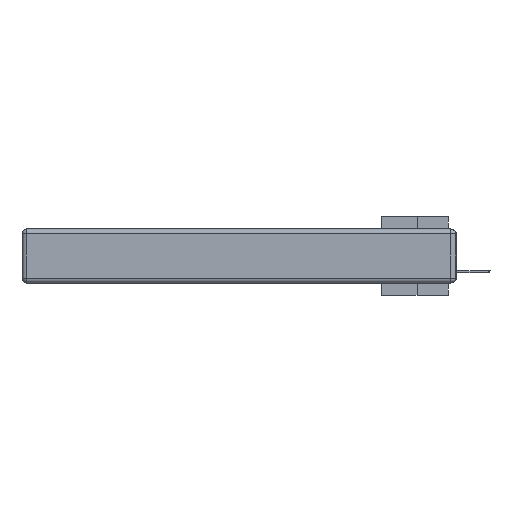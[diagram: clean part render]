
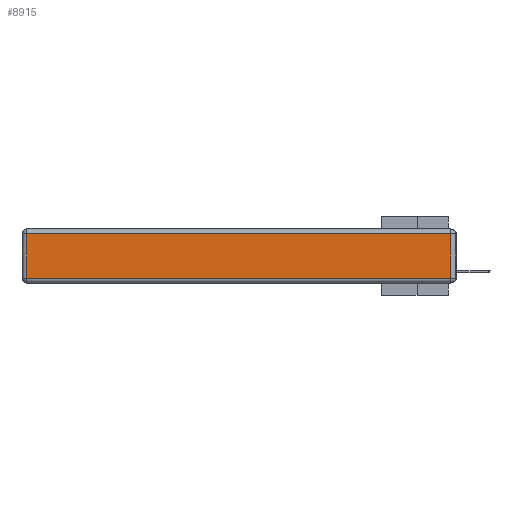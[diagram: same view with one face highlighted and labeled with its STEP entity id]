
A CAD part, left-side view. The second image highlights one B-rep face of the part: STEP entity #8915.
In plain terms, the highlighted planar face has unit normal (-1, 0, 0).
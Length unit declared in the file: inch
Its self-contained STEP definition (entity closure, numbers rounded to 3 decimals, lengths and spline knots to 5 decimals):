
#371 = AXIS2_PLACEMENT_3D ( 'NONE', #29806, #30139, #32342 ) ;
#604 = CARTESIAN_POINT ( 'NONE',  ( 0., 2.72, -0.313 ) ) ;
#1376 = VERTEX_POINT ( 'NONE', #10283 ) ;
#2145 = DIRECTION ( 'NONE',  ( 0., 0., -1. ) ) ;
#2337 = VECTOR ( 'NONE', #2145, 39.37008 ) ;
#3185 = LINE ( 'NONE', #16289, #25844 ) ;
#4667 = VERTEX_POINT ( 'NONE', #24505 ) ;
#5012 = CARTESIAN_POINT ( 'NONE',  ( 0., 0.03, -0.03 ) ) ;
#6037 = VERTEX_POINT ( 'NONE', #5012 ) ;
#6378 = EDGE_CURVE ( 'NONE', #6037, #4667, #3185, .T. ) ;
#8915 = ADVANCED_FACE ( 'NONE', ( #17005 ), #29910, .T. ) ;
#9785 = VERTEX_POINT ( 'NONE', #604 ) ;
#10283 = CARTESIAN_POINT ( 'NONE',  ( 0., 0.03, -0.313 ) ) ;
#13254 = EDGE_CURVE ( 'NONE', #9785, #1376, #29212, .T. ) ;
#13554 = EDGE_LOOP ( 'NONE', ( #20318, #16575, #25412, #30046 ) ) ;
#14306 = EDGE_CURVE ( 'NONE', #1376, #6037, #16960, .T. ) ;
#15090 = CARTESIAN_POINT ( 'NONE',  ( 0., 2.72, -0.343 ) ) ;
#16289 = CARTESIAN_POINT ( 'NONE',  ( 0., 2.75, -0.03 ) ) ;
#16575 = ORIENTED_EDGE ( 'NONE', *, *, #14306, .T. ) ;
#16960 = LINE ( 'NONE', #27470, #25617 ) ;
#17005 = FACE_OUTER_BOUND ( 'NONE', #13554, .T. ) ;
#19322 = DIRECTION ( 'NONE',  ( 0., 1., 0. ) ) ;
#20318 = ORIENTED_EDGE ( 'NONE', *, *, #13254, .T. ) ;
#21368 = EDGE_CURVE ( 'NONE', #4667, #9785, #21906, .T. ) ;
#21906 = LINE ( 'NONE', #15090, #2337 ) ;
#22531 = DIRECTION ( 'NONE',  ( 0., 0., 1. ) ) ;
#23252 = DIRECTION ( 'NONE',  ( 0., -1., 0. ) ) ;
#24505 = CARTESIAN_POINT ( 'NONE',  ( 0., 2.72, -0.03 ) ) ;
#25412 = ORIENTED_EDGE ( 'NONE', *, *, #6378, .T. ) ;
#25617 = VECTOR ( 'NONE', #22531, 39.37008 ) ;
#25646 = VECTOR ( 'NONE', #23252, 39.37008 ) ;
#25844 = VECTOR ( 'NONE', #19322, 39.37008 ) ;
#26174 = CARTESIAN_POINT ( 'NONE',  ( 0., 0., -0.313 ) ) ;
#27470 = CARTESIAN_POINT ( 'NONE',  ( 0., 0.03, -0.343 ) ) ;
#29212 = LINE ( 'NONE', #26174, #25646 ) ;
#29806 = CARTESIAN_POINT ( 'NONE',  ( 0., 0., -0.343 ) ) ;
#29910 = PLANE ( 'NONE',  #371 ) ;
#30046 = ORIENTED_EDGE ( 'NONE', *, *, #21368, .T. ) ;
#30139 = DIRECTION ( 'NONE',  ( -1., 0., 0. ) ) ;
#32342 = DIRECTION ( 'NONE',  ( 0., 0., 1. ) ) ;
